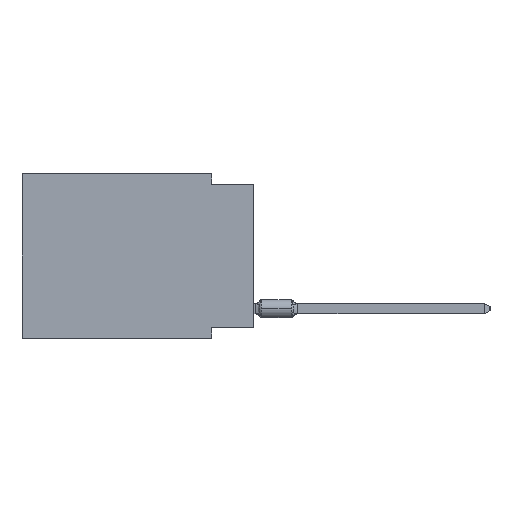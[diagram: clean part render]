
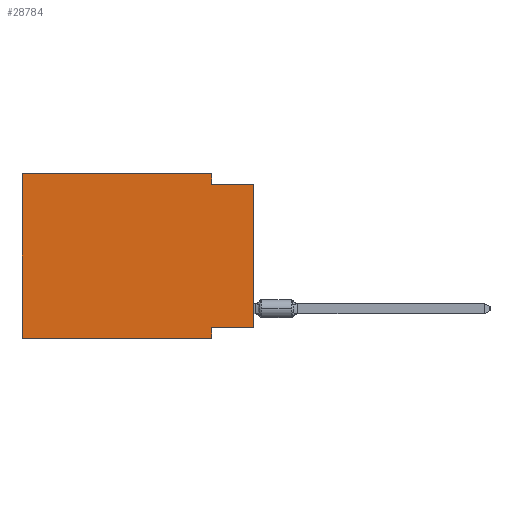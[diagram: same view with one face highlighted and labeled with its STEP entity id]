
A CAD part, left-side view. The second image highlights one B-rep face of the part: STEP entity #28784.
In plain terms, the highlighted planar face has unit normal (-1, 0, 0).
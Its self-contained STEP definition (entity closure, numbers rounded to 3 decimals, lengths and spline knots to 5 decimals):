
#1604 = LINE ( 'NONE', #62361, #63506 ) ;
#3366 = CARTESIAN_POINT ( 'NONE',  ( 0., 0., -0.025 ) ) ;
#3710 = CARTESIAN_POINT ( 'NONE',  ( 0., 0., -0.365 ) ) ;
#4520 = DIRECTION ( 'NONE',  ( 0., 0., -1. ) ) ;
#5431 = PLANE ( 'NONE',  #46295 ) ;
#5513 = EDGE_CURVE ( 'NONE', #22167, #47444, #12050, .T. ) ;
#8427 = VERTEX_POINT ( 'NONE', #25866 ) ;
#8725 = CARTESIAN_POINT ( 'NONE',  ( 0., 0.1, -0.365 ) ) ;
#10082 = VERTEX_POINT ( 'NONE', #8725 ) ;
#10470 = CARTESIAN_POINT ( 'NONE',  ( 0., 0.1, -0.39 ) ) ;
#12050 = LINE ( 'NONE', #53794, #18491 ) ;
#16106 = DIRECTION ( 'NONE',  ( 0., -1., 0. ) ) ;
#16474 = EDGE_CURVE ( 'NONE', #47444, #60290, #45594, .T. ) ;
#17753 = FACE_OUTER_BOUND ( 'NONE', #26957, .T. ) ;
#18491 = VECTOR ( 'NONE', #36304, 39.37008 ) ;
#20567 = LINE ( 'NONE', #33270, #33139 ) ;
#21532 = DIRECTION ( 'NONE',  ( 0., 0., 1. ) ) ;
#21907 = CARTESIAN_POINT ( 'NONE',  ( 0., 0.55, 0. ) ) ;
#22167 = VERTEX_POINT ( 'NONE', #21907 ) ;
#22422 = EDGE_CURVE ( 'NONE', #60091, #10082, #1604, .T. ) ;
#22659 = CARTESIAN_POINT ( 'NONE',  ( 0., 0.1, 0. ) ) ;
#22832 = EDGE_CURVE ( 'NONE', #61409, #22167, #20567, .T. ) ;
#25866 = CARTESIAN_POINT ( 'NONE',  ( 0., 0.1, -0.39 ) ) ;
#26084 = ORIENTED_EDGE ( 'NONE', *, *, #22832, .F. ) ;
#26957 = EDGE_LOOP ( 'NONE', ( #45111, #28078, #44375, #53934, #26084, #54872, #36554, #68327 ) ) ;
#28078 = ORIENTED_EDGE ( 'NONE', *, *, #66357, .F. ) ;
#28784 = ADVANCED_FACE ( 'NONE', ( #17753 ), #5431, .F. ) ;
#29673 = DIRECTION ( 'NONE',  ( 0., 0., -1. ) ) ;
#30295 = CARTESIAN_POINT ( 'NONE',  ( 0., 0.1, -0.025 ) ) ;
#32187 = DIRECTION ( 'NONE',  ( 0., 1., 0. ) ) ;
#33139 = VECTOR ( 'NONE', #44430, 39.37008 ) ;
#33270 = CARTESIAN_POINT ( 'NONE',  ( 0., 0.55, 0. ) ) ;
#33562 = LINE ( 'NONE', #3366, #42675 ) ;
#36304 = DIRECTION ( 'NONE',  ( 0., -1., 0. ) ) ;
#36409 = EDGE_CURVE ( 'NONE', #61409, #8427, #70491, .T. ) ;
#36554 = ORIENTED_EDGE ( 'NONE', *, *, #62414, .F. ) ;
#39523 = DIRECTION ( 'NONE',  ( 0., -1., 0. ) ) ;
#42675 = VECTOR ( 'NONE', #39523, 39.37008 ) ;
#43755 = VECTOR ( 'NONE', #4520, 39.37008 ) ;
#44375 = ORIENTED_EDGE ( 'NONE', *, *, #16474, .F. ) ;
#44430 = DIRECTION ( 'NONE',  ( 0., 0., 1. ) ) ;
#45111 = ORIENTED_EDGE ( 'NONE', *, *, #72531, .T. ) ;
#45594 = LINE ( 'NONE', #56736, #67477 ) ;
#46295 = AXIS2_PLACEMENT_3D ( 'NONE', #48340, #72546, #29673 ) ;
#47444 = VERTEX_POINT ( 'NONE', #22659 ) ;
#48340 = CARTESIAN_POINT ( 'NONE',  ( 0., 0.55, 0. ) ) ;
#49414 = VECTOR ( 'NONE', #16106, 39.37008 ) ;
#52654 = CARTESIAN_POINT ( 'NONE',  ( 0., 0.55, -0.39 ) ) ;
#53794 = CARTESIAN_POINT ( 'NONE',  ( 0., 0.55, 0. ) ) ;
#53934 = ORIENTED_EDGE ( 'NONE', *, *, #5513, .F. ) ;
#54872 = ORIENTED_EDGE ( 'NONE', *, *, #36409, .T. ) ;
#56736 = CARTESIAN_POINT ( 'NONE',  ( 0., 0.1, 0. ) ) ;
#58871 = LINE ( 'NONE', #71541, #73567 ) ;
#60091 = VERTEX_POINT ( 'NONE', #3710 ) ;
#60290 = VERTEX_POINT ( 'NONE', #30295 ) ;
#61409 = VERTEX_POINT ( 'NONE', #71212 ) ;
#62361 = CARTESIAN_POINT ( 'NONE',  ( 0., 0., -0.365 ) ) ;
#62414 = EDGE_CURVE ( 'NONE', #10082, #8427, #64884, .T. ) ;
#63506 = VECTOR ( 'NONE', #32187, 39.37008 ) ;
#64884 = LINE ( 'NONE', #10470, #43755 ) ;
#66357 = EDGE_CURVE ( 'NONE', #60290, #76334, #33562, .T. ) ;
#67477 = VECTOR ( 'NONE', #74577, 39.37008 ) ;
#68327 = ORIENTED_EDGE ( 'NONE', *, *, #22422, .F. ) ;
#69191 = CARTESIAN_POINT ( 'NONE',  ( 0., 0., -0.025 ) ) ;
#70491 = LINE ( 'NONE', #52654, #49414 ) ;
#71212 = CARTESIAN_POINT ( 'NONE',  ( 0., 0.55, -0.39 ) ) ;
#71541 = CARTESIAN_POINT ( 'NONE',  ( 0., 0., 0. ) ) ;
#72531 = EDGE_CURVE ( 'NONE', #60091, #76334, #58871, .T. ) ;
#72546 = DIRECTION ( 'NONE',  ( 1., 0., 0. ) ) ;
#73567 = VECTOR ( 'NONE', #21532, 39.37008 ) ;
#74577 = DIRECTION ( 'NONE',  ( 0., 0., -1. ) ) ;
#76334 = VERTEX_POINT ( 'NONE', #69191 ) ;
